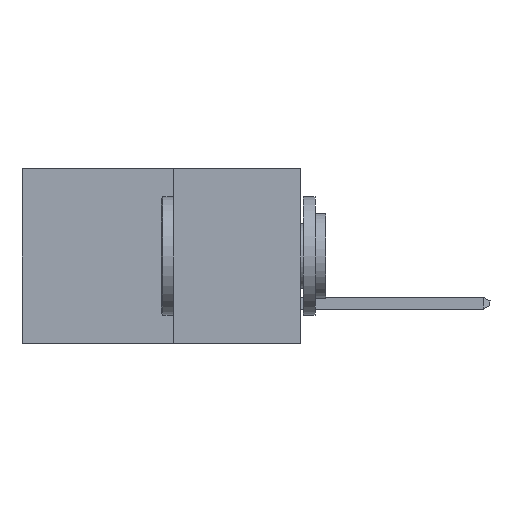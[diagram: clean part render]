
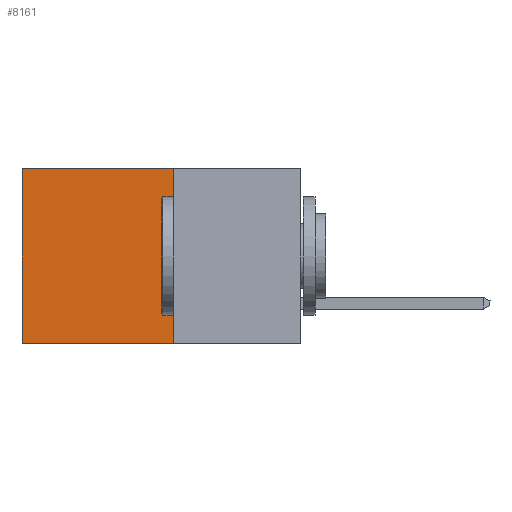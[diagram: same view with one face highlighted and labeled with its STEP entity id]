
A CAD part, left-side view. The second image highlights one B-rep face of the part: STEP entity #8161.
In plain terms, the highlighted planar face has unit normal (-1, 0, 0).
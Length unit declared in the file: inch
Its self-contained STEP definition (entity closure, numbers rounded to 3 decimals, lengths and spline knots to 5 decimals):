
#201 = EDGE_CURVE ( 'NONE', #13803, #18437, #13211, .T. ) ;
#1434 = LINE ( 'NONE', #9514, #13566 ) ;
#1508 = EDGE_CURVE ( 'NONE', #6817, #18559, #12169, .T. ) ;
#2329 = CARTESIAN_POINT ( 'NONE',  ( 0.277, 0.59, 0. ) ) ;
#2424 = VECTOR ( 'NONE', #25336, 39.37008 ) ;
#2877 = DIRECTION ( 'NONE',  ( 0., 1., 0. ) ) ;
#4120 = CARTESIAN_POINT ( 'NONE',  ( 0.277, 0.59, -0.37 ) ) ;
#4240 = CARTESIAN_POINT ( 'NONE',  ( 0.277, 0.27, -0.37 ) ) ;
#4487 = EDGE_CURVE ( 'NONE', #6817, #13803, #11903, .T. ) ;
#4739 = ORIENTED_EDGE ( 'NONE', *, *, #21901, .T. ) ;
#5126 = ORIENTED_EDGE ( 'NONE', *, *, #4487, .F. ) ;
#6152 = VECTOR ( 'NONE', #8527, 39.37008 ) ;
#6817 = VERTEX_POINT ( 'NONE', #18001 ) ;
#7343 = CARTESIAN_POINT ( 'NONE',  ( 0.277, 0.27, -0.37 ) ) ;
#8161 = ADVANCED_FACE ( 'NONE', ( #23734 ), #22660, .F. ) ;
#8527 = DIRECTION ( 'NONE',  ( 0., 0., -1. ) ) ;
#9514 = CARTESIAN_POINT ( 'NONE',  ( 0.277, 0.59, -0.37 ) ) ;
#11903 = LINE ( 'NONE', #7343, #6152 ) ;
#12169 = LINE ( 'NONE', #22925, #22854 ) ;
#13211 = LINE ( 'NONE', #20176, #2424 ) ;
#13566 = VECTOR ( 'NONE', #24452, 39.37008 ) ;
#13803 = VERTEX_POINT ( 'NONE', #4240 ) ;
#14140 = DIRECTION ( 'NONE',  ( 0., 0., -1. ) ) ;
#14476 = ORIENTED_EDGE ( 'NONE', *, *, #201, .F. ) ;
#18001 = CARTESIAN_POINT ( 'NONE',  ( 0.277, 0.27, 0. ) ) ;
#18437 = VERTEX_POINT ( 'NONE', #4120 ) ;
#18559 = VERTEX_POINT ( 'NONE', #2329 ) ;
#18891 = AXIS2_PLACEMENT_3D ( 'NONE', #24747, #26868, #14140 ) ;
#20176 = CARTESIAN_POINT ( 'NONE',  ( 0.277, 0.27, -0.37 ) ) ;
#20359 = EDGE_LOOP ( 'NONE', ( #4739, #14476, #5126, #21911 ) ) ;
#21901 = EDGE_CURVE ( 'NONE', #18559, #18437, #1434, .T. ) ;
#21911 = ORIENTED_EDGE ( 'NONE', *, *, #1508, .T. ) ;
#22660 = PLANE ( 'NONE',  #18891 ) ;
#22854 = VECTOR ( 'NONE', #2877, 39.37008 ) ;
#22925 = CARTESIAN_POINT ( 'NONE',  ( 0.277, 0.27, 0. ) ) ;
#23734 = FACE_OUTER_BOUND ( 'NONE', #20359, .T. ) ;
#24452 = DIRECTION ( 'NONE',  ( 0., 0., -1. ) ) ;
#24747 = CARTESIAN_POINT ( 'NONE',  ( 0.277, 0.27, -0.37 ) ) ;
#25336 = DIRECTION ( 'NONE',  ( 0., 1., 0. ) ) ;
#26868 = DIRECTION ( 'NONE',  ( 1., 0., 0. ) ) ;
